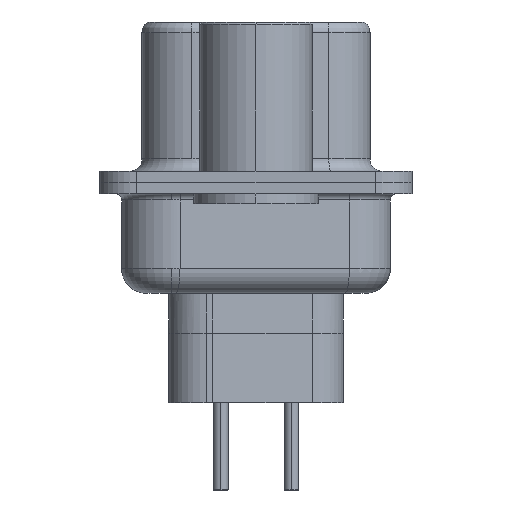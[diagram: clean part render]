
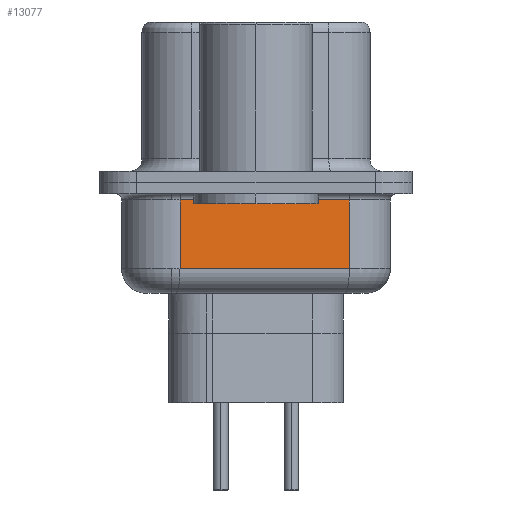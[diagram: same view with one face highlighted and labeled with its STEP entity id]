
A CAD part, left-side view. The second image highlights one B-rep face of the part: STEP entity #13077.
In plain terms, the highlighted planar face has unit normal (-0.985, -0.174, 0).
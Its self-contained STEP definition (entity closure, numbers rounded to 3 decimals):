
#613 = EDGE_CURVE ( 'NONE', #27140, #13683, #14363, .T. ) ;
#946 = DIRECTION ( 'NONE',  ( 0.985, 0.174, 0. ) ) ;
#958 = CARTESIAN_POINT ( 'NONE',  ( 4.049, -3.747, -0.7 ) ) ;
#1278 = LINE ( 'NONE', #9984, #7859 ) ;
#1406 = VECTOR ( 'NONE', #9387, 1000. ) ;
#1920 = CARTESIAN_POINT ( 'NONE',  ( 4.049, -3.747, -3.45 ) ) ;
#3887 = VERTEX_POINT ( 'NONE', #27741 ) ;
#4959 = CARTESIAN_POINT ( 'NONE',  ( 4.049, -3.747, -4.45 ) ) ;
#5122 = VECTOR ( 'NONE', #23622, 1000. ) ;
#5263 = DIRECTION ( 'NONE',  ( -0.174, 0.985, 0. ) ) ;
#6292 = AXIS2_PLACEMENT_3D ( 'NONE', #11920, #946, #7507 ) ;
#6381 = ORIENTED_EDGE ( 'NONE', *, *, #21219, .T. ) ;
#6469 = CARTESIAN_POINT ( 'NONE',  ( 2.85, 3.053, -0.7 ) ) ;
#7237 = LINE ( 'NONE', #4959, #1406 ) ;
#7507 = DIRECTION ( 'NONE',  ( -0.174, 0.985, 0. ) ) ;
#7859 = VECTOR ( 'NONE', #18641, 1000. ) ;
#8713 = LINE ( 'NONE', #15263, #5122 ) ;
#9387 = DIRECTION ( 'NONE',  ( 0., 0., 1. ) ) ;
#9984 = CARTESIAN_POINT ( 'NONE',  ( 2.85, 3.053, -4.45 ) ) ;
#11920 = CARTESIAN_POINT ( 'NONE',  ( 2.85, 3.053, -4.45 ) ) ;
#12547 = ORIENTED_EDGE ( 'NONE', *, *, #18454, .T. ) ;
#13077 = ADVANCED_FACE ( 'NONE', ( #27384 ), #22712, .F. ) ;
#13683 = VERTEX_POINT ( 'NONE', #6469 ) ;
#13813 = CARTESIAN_POINT ( 'NONE',  ( 2.85, 3.053, -0.7 ) ) ;
#14363 = LINE ( 'NONE', #13813, #26268 ) ;
#14647 = EDGE_LOOP ( 'NONE', ( #26677, #6381, #12547, #26390 ) ) ;
#15263 = CARTESIAN_POINT ( 'NONE',  ( 2.85, 3.053, -3.45 ) ) ;
#15880 = VERTEX_POINT ( 'NONE', #1920 ) ;
#18454 = EDGE_CURVE ( 'NONE', #15880, #27140, #7237, .T. ) ;
#18641 = DIRECTION ( 'NONE',  ( 0., 0., 1. ) ) ;
#21219 = EDGE_CURVE ( 'NONE', #3887, #15880, #8713, .T. ) ;
#21538 = EDGE_CURVE ( 'NONE', #3887, #13683, #1278, .T. ) ;
#22712 = PLANE ( 'NONE',  #6292 ) ;
#23622 = DIRECTION ( 'NONE',  ( 0.174, -0.985, 0. ) ) ;
#26268 = VECTOR ( 'NONE', #5263, 1000. ) ;
#26390 = ORIENTED_EDGE ( 'NONE', *, *, #613, .T. ) ;
#26677 = ORIENTED_EDGE ( 'NONE', *, *, #21538, .F. ) ;
#27140 = VERTEX_POINT ( 'NONE', #958 ) ;
#27384 = FACE_OUTER_BOUND ( 'NONE', #14647, .T. ) ;
#27741 = CARTESIAN_POINT ( 'NONE',  ( 2.85, 3.053, -3.45 ) ) ;
